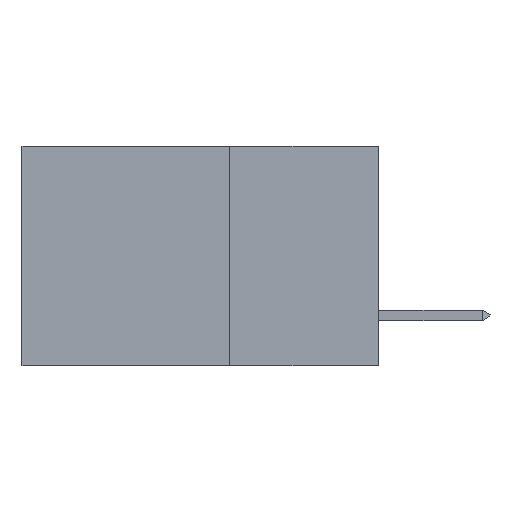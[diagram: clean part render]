
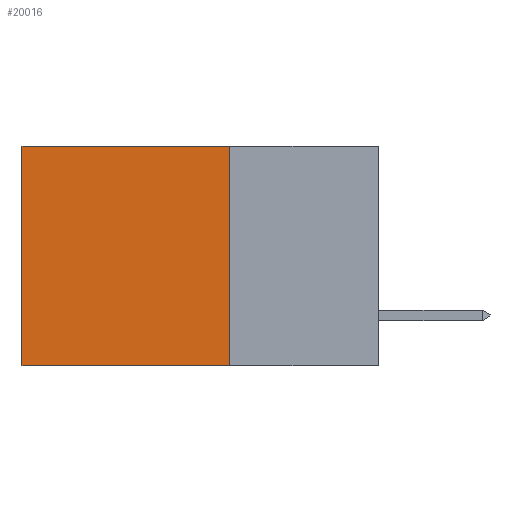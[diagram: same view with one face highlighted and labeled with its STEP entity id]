
A CAD part, left-side view. The second image highlights one B-rep face of the part: STEP entity #20016.
In plain terms, the highlighted planar face has unit normal (-1, 0, 0).
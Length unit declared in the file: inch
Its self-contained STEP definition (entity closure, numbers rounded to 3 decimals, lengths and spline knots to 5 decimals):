
#284 = DIRECTION ( 'NONE',  ( 1., 0., 0. ) ) ;
#1039 = EDGE_CURVE ( 'NONE', #17960, #12538, #21183, .T. ) ;
#1267 = EDGE_CURVE ( 'NONE', #17960, #21824, #21929, .T. ) ;
#2262 = CARTESIAN_POINT ( 'NONE',  ( 0.2615, 0.25, -0.37 ) ) ;
#3246 = ORIENTED_EDGE ( 'NONE', *, *, #8971, .T. ) ;
#3306 = EDGE_CURVE ( 'NONE', #21824, #15303, #15247, .T. ) ;
#4943 = DIRECTION ( 'NONE',  ( 0., 0., -1. ) ) ;
#5083 = CARTESIAN_POINT ( 'NONE',  ( 0.2615, 0.25, -0.37 ) ) ;
#6158 = DIRECTION ( 'NONE',  ( 0., 1., 0. ) ) ;
#6189 = ORIENTED_EDGE ( 'NONE', *, *, #1039, .T. ) ;
#8376 = CARTESIAN_POINT ( 'NONE',  ( 0.2615, 0.25, 0. ) ) ;
#8816 = VECTOR ( 'NONE', #14889, 39.37008 ) ;
#8971 = EDGE_CURVE ( 'NONE', #12538, #15303, #21452, .T. ) ;
#9229 = CARTESIAN_POINT ( 'NONE',  ( 0.2615, 0.25, -0.37 ) ) ;
#9454 = VECTOR ( 'NONE', #6158, 39.37008 ) ;
#11770 = CARTESIAN_POINT ( 'NONE',  ( 0.2615, 0.6, -0.37 ) ) ;
#12322 = CARTESIAN_POINT ( 'NONE',  ( 0.2615, 0.25, -0.37 ) ) ;
#12329 = CARTESIAN_POINT ( 'NONE',  ( 0.2615, 0.6, 0. ) ) ;
#12538 = VERTEX_POINT ( 'NONE', #12329 ) ;
#13938 = CARTESIAN_POINT ( 'NONE',  ( 0.2615, 0.6, -0.37 ) ) ;
#14504 = EDGE_LOOP ( 'NONE', ( #3246, #19308, #16023, #6189 ) ) ;
#14889 = DIRECTION ( 'NONE',  ( 0., 1., 0. ) ) ;
#15247 = LINE ( 'NONE', #9229, #8816 ) ;
#15303 = VERTEX_POINT ( 'NONE', #11770 ) ;
#15866 = CARTESIAN_POINT ( 'NONE',  ( 0.2615, 0.25, 0. ) ) ;
#16023 = ORIENTED_EDGE ( 'NONE', *, *, #1267, .F. ) ;
#17301 = PLANE ( 'NONE',  #22969 ) ;
#17960 = VERTEX_POINT ( 'NONE', #15866 ) ;
#19308 = ORIENTED_EDGE ( 'NONE', *, *, #3306, .F. ) ;
#19383 = DIRECTION ( 'NONE',  ( 0., 0., -1. ) ) ;
#19502 = VECTOR ( 'NONE', #23567, 39.37008 ) ;
#20016 = ADVANCED_FACE ( 'NONE', ( #22847 ), #17301, .F. ) ;
#21183 = LINE ( 'NONE', #8376, #9454 ) ;
#21452 = LINE ( 'NONE', #13938, #19502 ) ;
#21824 = VERTEX_POINT ( 'NONE', #5083 ) ;
#21929 = LINE ( 'NONE', #12322, #23254 ) ;
#22847 = FACE_OUTER_BOUND ( 'NONE', #14504, .T. ) ;
#22969 = AXIS2_PLACEMENT_3D ( 'NONE', #2262, #284, #19383 ) ;
#23254 = VECTOR ( 'NONE', #4943, 39.37008 ) ;
#23567 = DIRECTION ( 'NONE',  ( 0., 0., -1. ) ) ;
